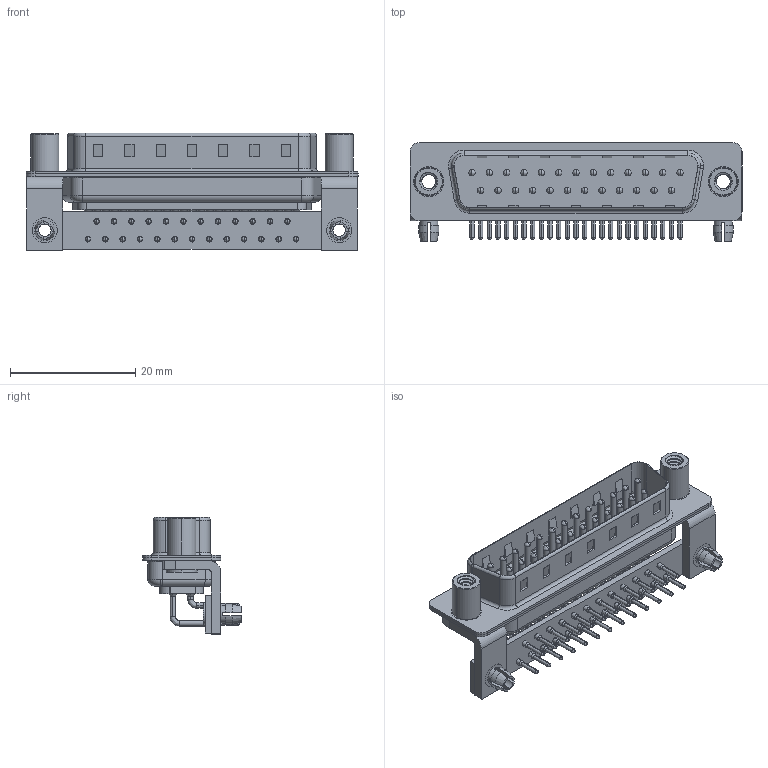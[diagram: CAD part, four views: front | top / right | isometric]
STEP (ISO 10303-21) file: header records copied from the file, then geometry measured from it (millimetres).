
FILE_DESCRIPTION (( 'STEP AP203' ), '1' );
FILE_NAME ('621-M25-360-LT5.STEP', '2018-09-25T03:41:10', ( '' ), ( '' ), 'SwSTEP 2.0', 'SolidWorks 2016', '' );
FILE_SCHEMA (( 'CONFIG_CONTROL_DESIGN' ));
Length unit declared in the file: millimetre
Products named in the file (10): 621M Shell Rear_25 Contacts; 621M Contact Row 1; 621M Contact Row 2; 621M Stabilizer Bracket; 621M 4-40 Threaded Standoff; 621M Stabilizer Board_25 Contacts; 621M Board Lock; 621M Housing_25 Contacts; 621-M25-360-LT5; 621M Shell Front_25 Contacts
Assembly tree (35 placements, depth 2):
  621-M25-360-LT5
    621M Housing_25 Contacts
    621M Shell Front_25 Contacts
    621M Shell Rear_25 Contacts
    621M Contact Row 1  x13
    621M Contact Row 2  x12
    621M Stabilizer Bracket  x2
    621M 4-40 Threaded Standoff  x2
    621M Stabilizer Board_25 Contacts
    621M Board Lock  x2
Bounding box: 53.05 x 15.8 x 18.8 mm (x, y, z)
Volume: 3557.5 mm3; surface area: 9450.4 mm2
Topology: 35 solids, 35 shells, 3368 faces, 9397 edges, 6116 vertices
Faces by surface type: plane 1847, cylinder 1183, bspline 156, cone 126, torus 56
Entity records: 31667 total; most frequent: CARTESIAN_POINT 6954, DIRECTION 5009, ORIENTED_EDGE 4646, EDGE_CURVE 2323, AXIS2_PLACEMENT_3D 1854, VERTEX_POINT 1509, VECTOR 1301, LINE 1301
